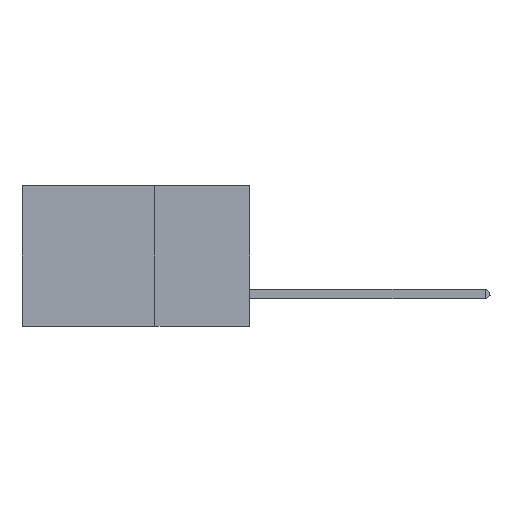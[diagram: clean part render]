
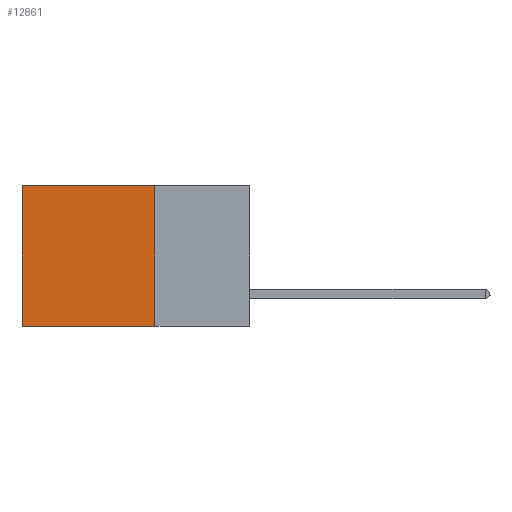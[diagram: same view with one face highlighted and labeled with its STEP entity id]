
A CAD part, left-side view. The second image highlights one B-rep face of the part: STEP entity #12861.
In plain terms, the highlighted planar face has unit normal (-1, 0, 0).
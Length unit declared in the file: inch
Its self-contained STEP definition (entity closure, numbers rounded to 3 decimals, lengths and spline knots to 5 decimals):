
#1090 = CARTESIAN_POINT ( 'NONE',  ( 0.2875, 0.25, 0. ) ) ;
#1684 = VERTEX_POINT ( 'NONE', #26405 ) ;
#1783 = CARTESIAN_POINT ( 'NONE',  ( 0.2875, 0.25, -0.37 ) ) ;
#3171 = EDGE_CURVE ( 'NONE', #1684, #11261, #24438, .T. ) ;
#3338 = LINE ( 'NONE', #30945, #11078 ) ;
#6811 = DIRECTION ( 'NONE',  ( 1., 0., 0. ) ) ;
#6874 = FACE_OUTER_BOUND ( 'NONE', #9216, .T. ) ;
#7031 = LINE ( 'NONE', #15819, #14825 ) ;
#7092 = PLANE ( 'NONE',  #20108 ) ;
#7266 = VERTEX_POINT ( 'NONE', #28515 ) ;
#8694 = CARTESIAN_POINT ( 'NONE',  ( 0.2875, 0.6, 0. ) ) ;
#9216 = EDGE_LOOP ( 'NONE', ( #13334, #12128, #23971, #25532 ) ) ;
#11078 = VECTOR ( 'NONE', #21022, 39.37008 ) ;
#11261 = VERTEX_POINT ( 'NONE', #8694 ) ;
#12128 = ORIENTED_EDGE ( 'NONE', *, *, #13484, .F. ) ;
#12861 = ADVANCED_FACE ( 'NONE', ( #6874 ), #7092, .F. ) ;
#13334 = ORIENTED_EDGE ( 'NONE', *, *, #18535, .T. ) ;
#13428 = DIRECTION ( 'NONE',  ( 0., 0., -1. ) ) ;
#13484 = EDGE_CURVE ( 'NONE', #20296, #7266, #18527, .T. ) ;
#13950 = EDGE_CURVE ( 'NONE', #1684, #20296, #3338, .T. ) ;
#14254 = VECTOR ( 'NONE', #22366, 39.37008 ) ;
#14825 = VECTOR ( 'NONE', #13428, 39.37008 ) ;
#15819 = CARTESIAN_POINT ( 'NONE',  ( 0.2875, 0.6, 0. ) ) ;
#16949 = DIRECTION ( 'NONE',  ( 0., 0., -1. ) ) ;
#18527 = LINE ( 'NONE', #20410, #14254 ) ;
#18535 = EDGE_CURVE ( 'NONE', #11261, #7266, #7031, .T. ) ;
#20108 = AXIS2_PLACEMENT_3D ( 'NONE', #1090, #6811, #16949 ) ;
#20296 = VERTEX_POINT ( 'NONE', #1783 ) ;
#20410 = CARTESIAN_POINT ( 'NONE',  ( 0.2875, 0.25, -0.37 ) ) ;
#21022 = DIRECTION ( 'NONE',  ( 0., 0., -1. ) ) ;
#22366 = DIRECTION ( 'NONE',  ( 0., 1., 0. ) ) ;
#23971 = ORIENTED_EDGE ( 'NONE', *, *, #13950, .F. ) ;
#24438 = LINE ( 'NONE', #25348, #31062 ) ;
#25348 = CARTESIAN_POINT ( 'NONE',  ( 0.2875, 0.25, 0. ) ) ;
#25532 = ORIENTED_EDGE ( 'NONE', *, *, #3171, .T. ) ;
#26405 = CARTESIAN_POINT ( 'NONE',  ( 0.2875, 0.25, 0. ) ) ;
#27320 = DIRECTION ( 'NONE',  ( 0., 1., 0. ) ) ;
#28515 = CARTESIAN_POINT ( 'NONE',  ( 0.2875, 0.6, -0.37 ) ) ;
#30945 = CARTESIAN_POINT ( 'NONE',  ( 0.2875, 0.25, 0. ) ) ;
#31062 = VECTOR ( 'NONE', #27320, 39.37008 ) ;
